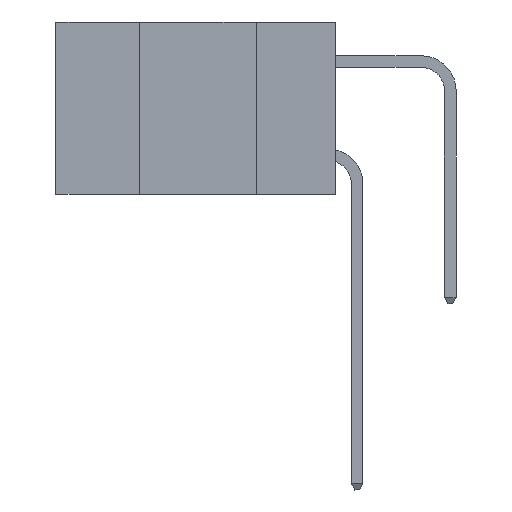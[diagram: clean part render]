
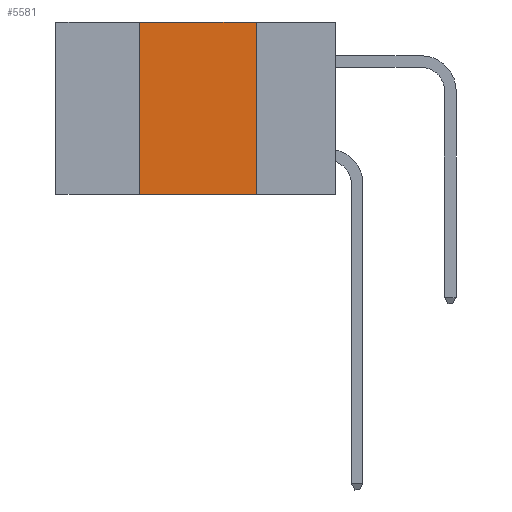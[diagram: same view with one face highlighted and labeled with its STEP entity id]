
A CAD part, left-side view. The second image highlights one B-rep face of the part: STEP entity #5581.
In plain terms, the highlighted planar face has unit normal (-1, 0, 0).
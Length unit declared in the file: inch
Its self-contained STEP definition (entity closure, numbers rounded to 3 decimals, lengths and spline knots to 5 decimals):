
#78 = VERTEX_POINT ( 'NONE', #5831 ) ;
#102 = EDGE_LOOP ( 'NONE', ( #6446, #560, #5385, #6904 ) ) ;
#127 = VECTOR ( 'NONE', #2776, 39.37008 ) ;
#560 = ORIENTED_EDGE ( 'NONE', *, *, #5208, .F. ) ;
#796 = VECTOR ( 'NONE', #6347, 39.37008 ) ;
#1155 = LINE ( 'NONE', #5932, #796 ) ;
#1458 = VECTOR ( 'NONE', #3362, 39.37008 ) ;
#2776 = DIRECTION ( 'NONE',  ( 0., -1., 0. ) ) ;
#2987 = DIRECTION ( 'NONE',  ( 0., 0., 1. ) ) ;
#3362 = DIRECTION ( 'NONE',  ( 0., -1., 0. ) ) ;
#4154 = CARTESIAN_POINT ( 'NONE',  ( 0., 0.6, -0.37 ) ) ;
#4357 = EDGE_CURVE ( 'NONE', #8872, #7766, #1155, .T. ) ;
#4375 = EDGE_CURVE ( 'NONE', #8431, #78, #7632, .T. ) ;
#4380 = EDGE_CURVE ( 'NONE', #8431, #7766, #9678, .T. ) ;
#4522 = PLANE ( 'NONE',  #10163 ) ;
#4552 = DIRECTION ( 'NONE',  ( 0., 0., -1. ) ) ;
#5084 = CARTESIAN_POINT ( 'NONE',  ( 0., 0.17, -0.37 ) ) ;
#5208 = EDGE_CURVE ( 'NONE', #78, #8872, #8822, .T. ) ;
#5385 = ORIENTED_EDGE ( 'NONE', *, *, #4375, .F. ) ;
#5415 = VECTOR ( 'NONE', #2987, 39.37008 ) ;
#5457 = CARTESIAN_POINT ( 'NONE',  ( 0., 0.6, 0. ) ) ;
#5581 = ADVANCED_FACE ( 'NONE', ( #9970 ), #4522, .F. ) ;
#5831 = CARTESIAN_POINT ( 'NONE',  ( 0., 0.42, 0. ) ) ;
#5873 = CARTESIAN_POINT ( 'NONE',  ( 0., 0.6, 0. ) ) ;
#5932 = CARTESIAN_POINT ( 'NONE',  ( 0., 0.17, 0. ) ) ;
#6347 = DIRECTION ( 'NONE',  ( 0., 0., -1. ) ) ;
#6446 = ORIENTED_EDGE ( 'NONE', *, *, #4357, .F. ) ;
#6904 = ORIENTED_EDGE ( 'NONE', *, *, #4380, .T. ) ;
#7556 = CARTESIAN_POINT ( 'NONE',  ( 0., 0.42, -0.37 ) ) ;
#7632 = LINE ( 'NONE', #11251, #5415 ) ;
#7766 = VERTEX_POINT ( 'NONE', #5084 ) ;
#8431 = VERTEX_POINT ( 'NONE', #7556 ) ;
#8822 = LINE ( 'NONE', #5873, #1458 ) ;
#8872 = VERTEX_POINT ( 'NONE', #9377 ) ;
#9377 = CARTESIAN_POINT ( 'NONE',  ( 0., 0.17, 0. ) ) ;
#9678 = LINE ( 'NONE', #4154, #127 ) ;
#9970 = FACE_OUTER_BOUND ( 'NONE', #102, .T. ) ;
#10163 = AXIS2_PLACEMENT_3D ( 'NONE', #5457, #10655, #4552 ) ;
#10655 = DIRECTION ( 'NONE',  ( 1., 0., 0. ) ) ;
#11251 = CARTESIAN_POINT ( 'NONE',  ( 0., 0.42, 0. ) ) ;
